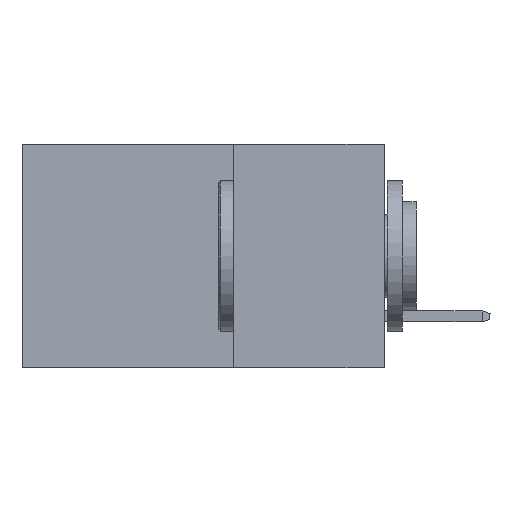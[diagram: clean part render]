
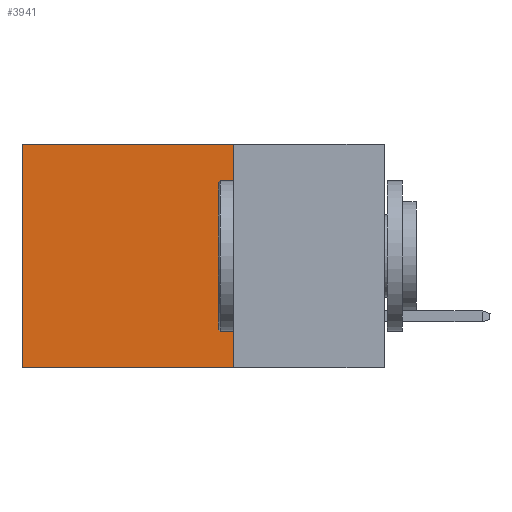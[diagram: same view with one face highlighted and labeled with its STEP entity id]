
A CAD part, left-side view. The second image highlights one B-rep face of the part: STEP entity #3941.
In plain terms, the highlighted planar face has unit normal (-1, 0, 0).
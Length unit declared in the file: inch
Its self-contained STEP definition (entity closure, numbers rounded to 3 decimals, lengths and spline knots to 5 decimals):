
#493 = EDGE_CURVE ( 'NONE', #7059, #11444, #12331, .T. ) ;
#497 = CARTESIAN_POINT ( 'NONE',  ( 0.2615, 0.6, -0.37 ) ) ;
#987 = DIRECTION ( 'NONE',  ( 0., 1., 0. ) ) ;
#1169 = VECTOR ( 'NONE', #4301, 39.37008 ) ;
#2702 = ORIENTED_EDGE ( 'NONE', *, *, #9444, .T. ) ;
#2712 = VERTEX_POINT ( 'NONE', #3219 ) ;
#2965 = EDGE_CURVE ( 'NONE', #2712, #11444, #11908, .T. ) ;
#3019 = VECTOR ( 'NONE', #6217, 39.37008 ) ;
#3051 = ORIENTED_EDGE ( 'NONE', *, *, #493, .T. ) ;
#3219 = CARTESIAN_POINT ( 'NONE',  ( 0.2615, 0.25, -0.37 ) ) ;
#3258 = CARTESIAN_POINT ( 'NONE',  ( 0.2615, 0.25, 0. ) ) ;
#3837 = VERTEX_POINT ( 'NONE', #3258 ) ;
#3913 = LINE ( 'NONE', #10128, #7501 ) ;
#3941 = ADVANCED_FACE ( 'NONE', ( #9604 ), #4826, .F. ) ;
#4107 = DIRECTION ( 'NONE',  ( 0., 0., -1. ) ) ;
#4221 = AXIS2_PLACEMENT_3D ( 'NONE', #5548, #8828, #5678 ) ;
#4301 = DIRECTION ( 'NONE',  ( 0., 0., -1. ) ) ;
#4826 = PLANE ( 'NONE',  #4221 ) ;
#5073 = CARTESIAN_POINT ( 'NONE',  ( 0.2615, 0.6, 0. ) ) ;
#5373 = EDGE_CURVE ( 'NONE', #3837, #2712, #3913, .T. ) ;
#5548 = CARTESIAN_POINT ( 'NONE',  ( 0.2615, 0.25, -0.37 ) ) ;
#5678 = DIRECTION ( 'NONE',  ( 0., 0., -1. ) ) ;
#6217 = DIRECTION ( 'NONE',  ( 0., 1., 0. ) ) ;
#6282 = LINE ( 'NONE', #11305, #3019 ) ;
#7059 = VERTEX_POINT ( 'NONE', #5073 ) ;
#7501 = VECTOR ( 'NONE', #4107, 39.37008 ) ;
#8828 = DIRECTION ( 'NONE',  ( 1., 0., 0. ) ) ;
#9444 = EDGE_CURVE ( 'NONE', #3837, #7059, #6282, .T. ) ;
#9604 = FACE_OUTER_BOUND ( 'NONE', #11012, .T. ) ;
#10042 = CARTESIAN_POINT ( 'NONE',  ( 0.2615, 0.6, -0.37 ) ) ;
#10082 = CARTESIAN_POINT ( 'NONE',  ( 0.2615, 0.25, -0.37 ) ) ;
#10128 = CARTESIAN_POINT ( 'NONE',  ( 0.2615, 0.25, -0.37 ) ) ;
#10236 = VECTOR ( 'NONE', #987, 39.37008 ) ;
#10632 = ORIENTED_EDGE ( 'NONE', *, *, #5373, .F. ) ;
#11012 = EDGE_LOOP ( 'NONE', ( #3051, #11517, #10632, #2702 ) ) ;
#11305 = CARTESIAN_POINT ( 'NONE',  ( 0.2615, 0.25, 0. ) ) ;
#11444 = VERTEX_POINT ( 'NONE', #10042 ) ;
#11517 = ORIENTED_EDGE ( 'NONE', *, *, #2965, .F. ) ;
#11908 = LINE ( 'NONE', #10082, #10236 ) ;
#12331 = LINE ( 'NONE', #497, #1169 ) ;
